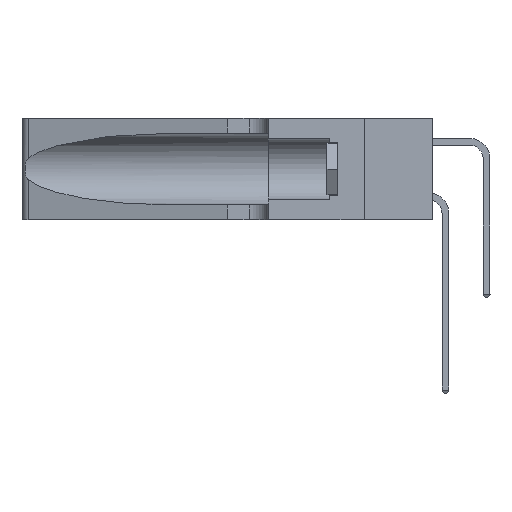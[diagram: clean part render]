
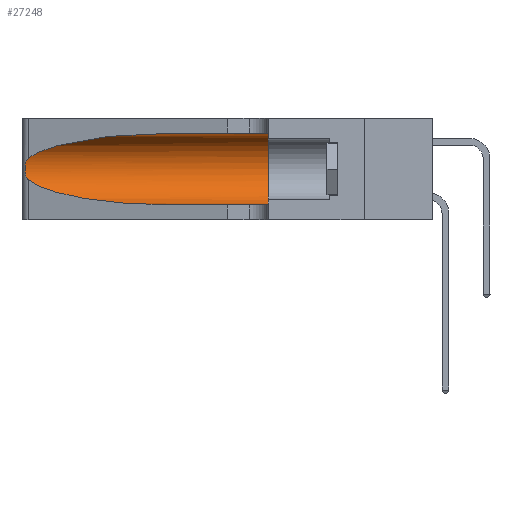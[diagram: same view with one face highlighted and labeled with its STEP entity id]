
A CAD part, left-side view. The second image highlights one B-rep face of the part: STEP entity #27248.
In plain terms, the highlighted cylindrical face has radius 3.308 mm (diameter 6.617 mm), a partial arc.
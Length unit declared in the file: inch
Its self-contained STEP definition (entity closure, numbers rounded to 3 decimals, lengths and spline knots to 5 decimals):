
#696 = VECTOR ( 'NONE', #39829, 39.37008 ) ;
#971 = VERTEX_POINT ( 'NONE', #38479 ) ;
#1716 = EDGE_LOOP ( 'NONE', ( #25957, #18881, #29237, #25678, #11475, #31174 ) ) ;
#2695 = CARTESIAN_POINT ( 'NONE',  ( 0.26075, 1.23896, 0.19203 ) ) ;
#2759 = CARTESIAN_POINT ( 'NONE',  ( 0.1305, 1.61858, 0.05475 ) ) ;
#4008 = CARTESIAN_POINT ( 'NONE',  ( 0.25789, 1.23486, 0.15765 ) ) ;
#4832 = EDGE_CURVE ( 'NONE', #971, #16222, #27096, .T. ) ;
#7282 = DIRECTION ( 'NONE',  ( 0., -1., 0. ) ) ;
#7594 = VECTOR ( 'NONE', #19298, 39.37008 ) ;
#7921 = CARTESIAN_POINT ( 'NONE',  ( 0.25639, 1.23184, 0.21858 ) ) ;
#8514 = CARTESIAN_POINT ( 'NONE',  ( 0.25639, 1.23186, 0.15144 ) ) ;
#8608 = CARTESIAN_POINT ( 'NONE',  ( 0.25487, 1.22718, 0.22369 ) ) ;
#8992 = CARTESIAN_POINT ( 'NONE',  ( 0.25487, 1.22718, 0.22369 ) ) ;
#10789 = EDGE_CURVE ( 'NONE', #24863, #971, #38658, .T. ) ;
#11475 = ORIENTED_EDGE ( 'NONE', *, *, #24221, .F. ) ;
#11968 = CARTESIAN_POINT ( 'NONE',  ( 0.25787, 1.23484, 0.2124 ) ) ;
#12486 = CARTESIAN_POINT ( 'NONE',  ( 0.26075, 1.23896, 0.178 ) ) ;
#12661 = CARTESIAN_POINT ( 'NONE',  ( 0.25487, 1.22718, 0.22369 ) ) ;
#12788 = VERTEX_POINT ( 'NONE', #36814 ) ;
#12852 = CIRCLE ( 'NONE', #35383, 0.13025 ) ;
#13247 = CARTESIAN_POINT ( 'NONE',  ( 0.1305, 0.35, 0.05475 ) ) ;
#14410 = CARTESIAN_POINT ( 'NONE',  ( 0.1305, 0.35, 0.185 ) ) ;
#15081 = EDGE_CURVE ( 'NONE', #38387, #24863, #18857, .T. ) ;
#15315 = CARTESIAN_POINT ( 'NONE',  ( 0.25854, 1.2359, 0.20912 ) ) ;
#15732 = CARTESIAN_POINT ( 'NONE',  ( 0.26017, 1.23833, 0.17102 ) ) ;
#15885 = CARTESIAN_POINT ( 'NONE',  ( 0.25487, 1.22718, 0.14631 ) ) ;
#16222 = VERTEX_POINT ( 'NONE', #13247 ) ;
#16776 = CARTESIAN_POINT ( 'NONE',  ( 0.25487, 1.22718, 0.14631 ) ) ;
#16935 = EDGE_CURVE ( 'NONE', #26099, #12788, #41230, .T. ) ;
#18042 = DIRECTION ( 'NONE',  ( 0., 1., 0. ) ) ;
#18343 = CARTESIAN_POINT ( 'NONE',  ( 0.1305, 1.61858, 0.185 ) ) ;
#18372 = CARTESIAN_POINT ( 'NONE',  ( 0.1305, 0.72297, 0.05475 ) ) ;
#18857 = B_SPLINE_CURVE_WITH_KNOTS ( 'NONE', 3,
 ( #8992, #41231, #7921, #11968, #15315, #28187, #2695, #12486, #15732, #28993, #4008, #8514, #37462, #40952 ),
 .UNSPECIFIED., .F., .F.,
 ( 4, 2, 2, 2, 2, 2, 4 ),
 ( 0., 0.00027, 0.00053, 0.00107, 0.0016, 0.00187, 0.00214 ),
 .UNSPECIFIED. ) ;
#18881 = ORIENTED_EDGE ( 'NONE', *, *, #15081, .T. ) ;
#19006 = AXIS2_PLACEMENT_3D ( 'NONE', #18343, #7282, #38702 ) ;
#19298 = DIRECTION ( 'NONE',  ( 0., -1., 0. ) ) ;
#23706 = CARTESIAN_POINT ( 'NONE',  ( 0.18966, 0.96281, 0.31525 ) ) ;
#24221 = EDGE_CURVE ( 'NONE', #12788, #16222, #12852, .T. ) ;
#24863 = VERTEX_POINT ( 'NONE', #16776 ) ;
#24986 = CARTESIAN_POINT ( 'NONE',  ( 0.2373, 1.15595, 0.28018 ) ) ;
#25196 = CYLINDRICAL_SURFACE ( 'NONE', #19006, 0.13025 ) ;
#25678 = ORIENTED_EDGE ( 'NONE', *, *, #4832, .T. ) ;
#25957 = ORIENTED_EDGE ( 'NONE', *, *, #38924, .T. ) ;
#26099 = VERTEX_POINT ( 'NONE', #34558 ) ;
#27043 =( BOUNDED_CURVE ( )  B_SPLINE_CURVE ( 3, ( #27202, #23706, #24986, #8608 ),
 .UNSPECIFIED., .F., .T. ) 
 B_SPLINE_CURVE_WITH_KNOTS ( ( 4, 4 ),
 ( 1.5708, 2.84003 ),
 .UNSPECIFIED. ) 
 CURVE ( )  GEOMETRIC_REPRESENTATION_ITEM ( )  RATIONAL_B_SPLINE_CURVE ( ( 1., 0.87, 0.87, 1. ) ) 
 REPRESENTATION_ITEM ( '' )  );
#27057 = CARTESIAN_POINT ( 'NONE',  ( 0.2373, 1.15595, 0.08982 ) ) ;
#27096 = LINE ( 'NONE', #2759, #7594 ) ;
#27202 = CARTESIAN_POINT ( 'NONE',  ( 0.1305, 0.72297, 0.31525 ) ) ;
#27248 = ADVANCED_FACE ( 'NONE', ( #32103 ), #25196, .F. ) ;
#28187 = CARTESIAN_POINT ( 'NONE',  ( 0.26018, 1.23835, 0.19895 ) ) ;
#28993 = CARTESIAN_POINT ( 'NONE',  ( 0.25856, 1.23593, 0.16098 ) ) ;
#29237 = ORIENTED_EDGE ( 'NONE', *, *, #10789, .T. ) ;
#30242 = CARTESIAN_POINT ( 'NONE',  ( 0.18966, 0.96281, 0.05475 ) ) ;
#31174 = ORIENTED_EDGE ( 'NONE', *, *, #16935, .F. ) ;
#32103 = FACE_OUTER_BOUND ( 'NONE', #1716, .T. ) ;
#33512 = DIRECTION ( 'NONE',  ( 0., 0., 1. ) ) ;
#34558 = CARTESIAN_POINT ( 'NONE',  ( 0.1305, 0.72297, 0.31525 ) ) ;
#35383 = AXIS2_PLACEMENT_3D ( 'NONE', #14410, #18042, #33512 ) ;
#36814 = CARTESIAN_POINT ( 'NONE',  ( 0.1305, 0.35, 0.31525 ) ) ;
#37319 = CARTESIAN_POINT ( 'NONE',  ( 0.1305, 1.61858, 0.31525 ) ) ;
#37462 = CARTESIAN_POINT ( 'NONE',  ( 0.25555, 1.22993, 0.14849 ) ) ;
#38387 = VERTEX_POINT ( 'NONE', #12661 ) ;
#38479 = CARTESIAN_POINT ( 'NONE',  ( 0.1305, 0.72297, 0.05475 ) ) ;
#38658 =( BOUNDED_CURVE ( )  B_SPLINE_CURVE ( 3, ( #15885, #27057, #30242, #18372 ),
 .UNSPECIFIED., .F., .T. ) 
 B_SPLINE_CURVE_WITH_KNOTS ( ( 4, 4 ),
 ( 3.44316, 4.71239 ),
 .UNSPECIFIED. ) 
 CURVE ( )  GEOMETRIC_REPRESENTATION_ITEM ( )  RATIONAL_B_SPLINE_CURVE ( ( 1., 0.87, 0.87, 1. ) ) 
 REPRESENTATION_ITEM ( '' )  );
#38702 = DIRECTION ( 'NONE',  ( 0., 0., -1. ) ) ;
#38924 = EDGE_CURVE ( 'NONE', #26099, #38387, #27043, .T. ) ;
#39829 = DIRECTION ( 'NONE',  ( 0., -1., 0. ) ) ;
#40952 = CARTESIAN_POINT ( 'NONE',  ( 0.25487, 1.22718, 0.14631 ) ) ;
#41230 = LINE ( 'NONE', #37319, #696 ) ;
#41231 = CARTESIAN_POINT ( 'NONE',  ( 0.25555, 1.22994, 0.2215 ) ) ;
